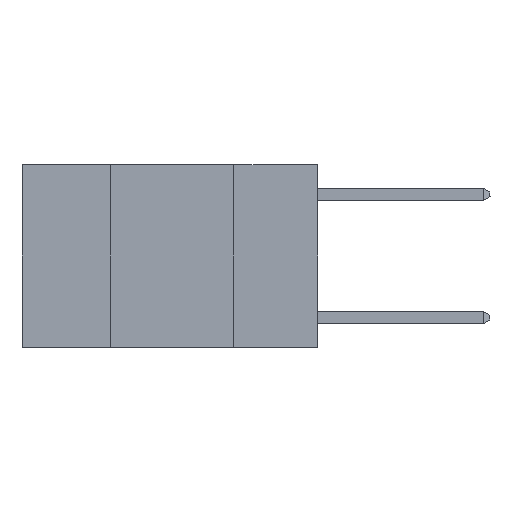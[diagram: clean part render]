
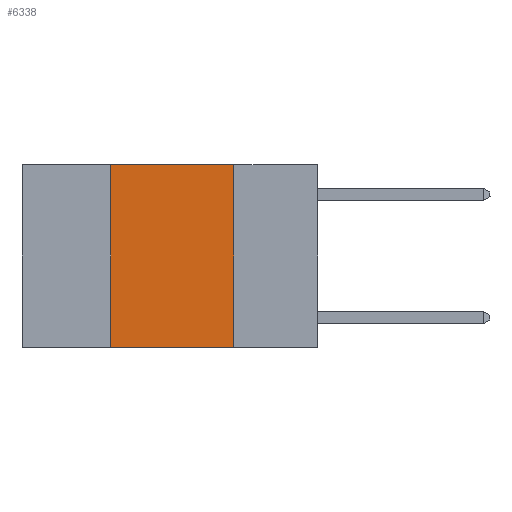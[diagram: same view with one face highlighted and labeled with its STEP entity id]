
A CAD part, left-side view. The second image highlights one B-rep face of the part: STEP entity #6338.
In plain terms, the highlighted planar face has unit normal (-1, 0, 0).
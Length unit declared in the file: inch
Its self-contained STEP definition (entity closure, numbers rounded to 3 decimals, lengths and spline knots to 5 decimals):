
#49 = VERTEX_POINT ( 'NONE', #4438 ) ;
#297 = DIRECTION ( 'NONE',  ( 0., -1., 0. ) ) ;
#436 = CARTESIAN_POINT ( 'NONE',  ( 0., 0.17, 0. ) ) ;
#1498 = DIRECTION ( 'NONE',  ( 0., -1., 0. ) ) ;
#1596 = LINE ( 'NONE', #3073, #8707 ) ;
#1641 = EDGE_CURVE ( 'NONE', #6945, #3514, #7631, .T. ) ;
#1653 = LINE ( 'NONE', #5835, #5609 ) ;
#1664 = CARTESIAN_POINT ( 'NONE',  ( 0., 0.17, 0. ) ) ;
#1997 = DIRECTION ( 'NONE',  ( 1., 0., 0. ) ) ;
#2251 = VERTEX_POINT ( 'NONE', #436 ) ;
#2520 = CARTESIAN_POINT ( 'NONE',  ( 0., 0.6, 0. ) ) ;
#3073 = CARTESIAN_POINT ( 'NONE',  ( 0., 0.42, 0. ) ) ;
#3432 = CARTESIAN_POINT ( 'NONE',  ( 0., 0.42, -0.37 ) ) ;
#3461 = AXIS2_PLACEMENT_3D ( 'NONE', #2520, #1997, #5328 ) ;
#3514 = VERTEX_POINT ( 'NONE', #5181 ) ;
#4438 = CARTESIAN_POINT ( 'NONE',  ( 0., 0.42, 0. ) ) ;
#4668 = PLANE ( 'NONE',  #3461 ) ;
#4872 = EDGE_CURVE ( 'NONE', #6945, #49, #1596, .T. ) ;
#4946 = CARTESIAN_POINT ( 'NONE',  ( 0., 0.6, -0.37 ) ) ;
#5181 = CARTESIAN_POINT ( 'NONE',  ( 0., 0.17, -0.37 ) ) ;
#5328 = DIRECTION ( 'NONE',  ( 0., 0., -1. ) ) ;
#5470 = FACE_OUTER_BOUND ( 'NONE', #6082, .T. ) ;
#5609 = VECTOR ( 'NONE', #297, 39.37008 ) ;
#5787 = EDGE_CURVE ( 'NONE', #49, #2251, #1653, .T. ) ;
#5792 = DIRECTION ( 'NONE',  ( 0., 0., 1. ) ) ;
#5835 = CARTESIAN_POINT ( 'NONE',  ( 0., 0.6, 0. ) ) ;
#6082 = EDGE_LOOP ( 'NONE', ( #7250, #6585, #8487, #7718 ) ) ;
#6338 = ADVANCED_FACE ( 'NONE', ( #5470 ), #4668, .F. ) ;
#6585 = ORIENTED_EDGE ( 'NONE', *, *, #5787, .F. ) ;
#6945 = VERTEX_POINT ( 'NONE', #3432 ) ;
#7144 = DIRECTION ( 'NONE',  ( 0., 0., -1. ) ) ;
#7250 = ORIENTED_EDGE ( 'NONE', *, *, #8368, .F. ) ;
#7594 = VECTOR ( 'NONE', #1498, 39.37008 ) ;
#7631 = LINE ( 'NONE', #4946, #7594 ) ;
#7718 = ORIENTED_EDGE ( 'NONE', *, *, #1641, .T. ) ;
#7793 = LINE ( 'NONE', #1664, #7888 ) ;
#7888 = VECTOR ( 'NONE', #7144, 39.37008 ) ;
#8368 = EDGE_CURVE ( 'NONE', #2251, #3514, #7793, .T. ) ;
#8487 = ORIENTED_EDGE ( 'NONE', *, *, #4872, .F. ) ;
#8707 = VECTOR ( 'NONE', #5792, 39.37008 ) ;
